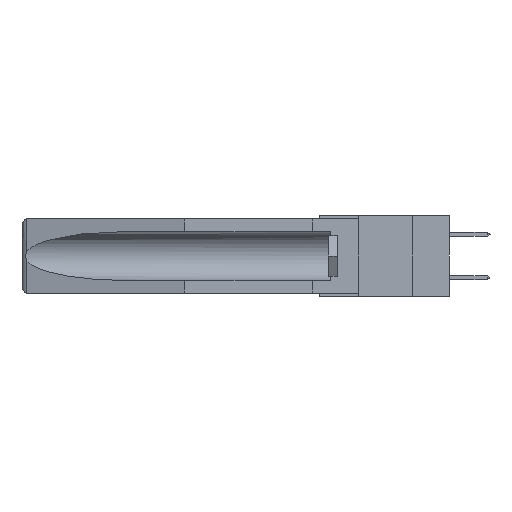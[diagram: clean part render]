
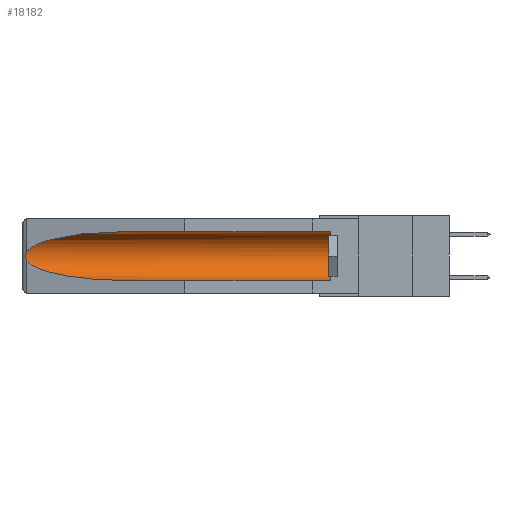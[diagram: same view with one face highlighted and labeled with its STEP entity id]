
A CAD part, left-side view. The second image highlights one B-rep face of the part: STEP entity #18182.
In plain terms, the highlighted cylindrical face has radius 2.857 mm (diameter 5.715 mm), a partial arc.
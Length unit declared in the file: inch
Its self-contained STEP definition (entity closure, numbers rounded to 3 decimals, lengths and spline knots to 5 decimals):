
#367 = ORIENTED_EDGE ( 'NONE', *, *, #15120, .T. ) ;
#2847 = LINE ( 'NONE', #16621, #24788 ) ;
#3473 = VERTEX_POINT ( 'NONE', #22331 ) ;
#3673 = EDGE_CURVE ( 'NONE', #22735, #22825, #7469, .T. ) ;
#3933 = CARTESIAN_POINT ( 'NONE',  ( 0.155, 0.126, -0.059 ) ) ;
#4370 = CARTESIAN_POINT ( 'NONE',  ( 0.155, 1.07973, -0.284 ) ) ;
#5345 = CARTESIAN_POINT ( 'NONE',  ( 0.26537, 1.52718, -0.19328 ) ) ;
#5605 = AXIS2_PLACEMENT_3D ( 'NONE', #23266, #19071, #17118 ) ;
#5941 = DIRECTION ( 'NONE',  ( 0., 1., 0. ) ) ;
#6650 = B_SPLINE_CURVE_WITH_KNOTS ( 'NONE', 3,
 ( #11245, #21569, #26173, #9099, #17680, #6893, #13090, #9195, #11066, #13365 ),
 .UNSPECIFIED., .F., .F.,
 ( 4, 2, 2, 2, 4 ),
 ( 0., 0.00029, 0.00058, 0.00087, 0.00117 ),
 .UNSPECIFIED. ) ;
#6893 = CARTESIAN_POINT ( 'NONE',  ( 0.2675, 1.53308, -0.17534 ) ) ;
#7223 = CYLINDRICAL_SURFACE ( 'NONE', #5605, 0.1125 ) ;
#7469 =( BOUNDED_CURVE ( )  B_SPLINE_CURVE ( 3, ( #10712, #19004, #23375, #14985 ),
 .UNSPECIFIED., .F., .F. ) 
 B_SPLINE_CURVE_WITH_KNOTS ( ( 4, 4 ),
 ( 4.71239, 6.08839 ),
 .UNSPECIFIED. ) 
 CURVE ( )  GEOMETRIC_REPRESENTATION_ITEM ( )  RATIONAL_B_SPLINE_CURVE ( ( 1., 0.848, 0.848, 1. ) ) 
 REPRESENTATION_ITEM ( '' )  );
#7756 = VERTEX_POINT ( 'NONE', #3933 ) ;
#8251 = EDGE_CURVE ( 'NONE', #7756, #22735, #2847, .T. ) ;
#8991 = EDGE_CURVE ( 'NONE', #22825, #3473, #6650, .T. ) ;
#9099 = CARTESIAN_POINT ( 'NONE',  ( 0.2673, 1.5327, -0.16383 ) ) ;
#9195 = CARTESIAN_POINT ( 'NONE',  ( 0.26655, 1.53094, -0.18657 ) ) ;
#10554 = ORIENTED_EDGE ( 'NONE', *, *, #3673, .T. ) ;
#10712 = CARTESIAN_POINT ( 'NONE',  ( 0.155, 1.07973, -0.059 ) ) ;
#11066 = CARTESIAN_POINT ( 'NONE',  ( 0.26597, 1.5296, -0.19026 ) ) ;
#11245 = CARTESIAN_POINT ( 'NONE',  ( 0.26537, 1.52718, -0.14972 ) ) ;
#12961 = EDGE_LOOP ( 'NONE', ( #10554, #13320, #367, #12995, #19176, #27422 ) ) ;
#12995 = ORIENTED_EDGE ( 'NONE', *, *, #15663, .F. ) ;
#13090 = CARTESIAN_POINT ( 'NONE',  ( 0.2673, 1.53269, -0.17917 ) ) ;
#13320 = ORIENTED_EDGE ( 'NONE', *, *, #8991, .T. ) ;
#13365 = CARTESIAN_POINT ( 'NONE',  ( 0.26537, 1.52718, -0.19328 ) ) ;
#13587 = DIRECTION ( 'NONE',  ( 0., -1., 0. ) ) ;
#13748 = CARTESIAN_POINT ( 'NONE',  ( 0.21114, 1.30732, -0.284 ) ) ;
#14320 = DIRECTION ( 'NONE',  ( 0., 1., 0. ) ) ;
#14541 = CARTESIAN_POINT ( 'NONE',  ( 0.155, 1.07973, -0.059 ) ) ;
#14985 = CARTESIAN_POINT ( 'NONE',  ( 0.26537, 1.52718, -0.14972 ) ) ;
#15120 = EDGE_CURVE ( 'NONE', #3473, #26263, #18226, .T. ) ;
#15663 = EDGE_CURVE ( 'NONE', #26857, #26263, #24049, .T. ) ;
#15803 = CARTESIAN_POINT ( 'NONE',  ( 0.25451, 1.48313, -0.24835 ) ) ;
#16184 = CIRCLE ( 'NONE', #21618, 0.1125 ) ;
#16621 = CARTESIAN_POINT ( 'NONE',  ( 0.155, -0.30754, -0.059 ) ) ;
#17118 = DIRECTION ( 'NONE',  ( 0., 0., 1. ) ) ;
#17680 = CARTESIAN_POINT ( 'NONE',  ( 0.2675, 1.53308, -0.16763 ) ) ;
#18182 = ADVANCED_FACE ( 'NONE', ( #26260 ), #7223, .F. ) ;
#18226 =( BOUNDED_CURVE ( )  B_SPLINE_CURVE ( 3, ( #5345, #15803, #13748, #20175 ),
 .UNSPECIFIED., .F., .T. ) 
 B_SPLINE_CURVE_WITH_KNOTS ( ( 4, 4 ),
 ( 0.1948, 1.5708 ),
 .UNSPECIFIED. ) 
 CURVE ( )  GEOMETRIC_REPRESENTATION_ITEM ( )  RATIONAL_B_SPLINE_CURVE ( ( 1., 0.848, 0.848, 1. ) ) 
 REPRESENTATION_ITEM ( '' )  );
#18388 = VECTOR ( 'NONE', #14320, 39.37008 ) ;
#18502 = EDGE_CURVE ( 'NONE', #26857, #7756, #16184, .T. ) ;
#19004 = CARTESIAN_POINT ( 'NONE',  ( 0.21114, 1.30732, -0.059 ) ) ;
#19071 = DIRECTION ( 'NONE',  ( 0., 1., 0. ) ) ;
#19176 = ORIENTED_EDGE ( 'NONE', *, *, #18502, .T. ) ;
#20175 = CARTESIAN_POINT ( 'NONE',  ( 0.155, 1.07973, -0.284 ) ) ;
#20975 = CARTESIAN_POINT ( 'NONE',  ( 0.155, -0.30754, -0.284 ) ) ;
#21217 = CARTESIAN_POINT ( 'NONE',  ( 0.26537, 1.52718, -0.14972 ) ) ;
#21569 = CARTESIAN_POINT ( 'NONE',  ( 0.26597, 1.52961, -0.15275 ) ) ;
#21618 = AXIS2_PLACEMENT_3D ( 'NONE', #24516, #13587, #24324 ) ;
#22331 = CARTESIAN_POINT ( 'NONE',  ( 0.26537, 1.52718, -0.19328 ) ) ;
#22735 = VERTEX_POINT ( 'NONE', #14541 ) ;
#22825 = VERTEX_POINT ( 'NONE', #21217 ) ;
#23266 = CARTESIAN_POINT ( 'NONE',  ( 0.155, -0.30754, -0.1715 ) ) ;
#23375 = CARTESIAN_POINT ( 'NONE',  ( 0.25451, 1.48313, -0.09465 ) ) ;
#24049 = LINE ( 'NONE', #20975, #18388 ) ;
#24324 = DIRECTION ( 'NONE',  ( 0., 0., 1. ) ) ;
#24516 = CARTESIAN_POINT ( 'NONE',  ( 0.155, 0.126, -0.1715 ) ) ;
#24788 = VECTOR ( 'NONE', #5941, 39.37008 ) ;
#26173 = CARTESIAN_POINT ( 'NONE',  ( 0.26654, 1.53092, -0.15636 ) ) ;
#26260 = FACE_OUTER_BOUND ( 'NONE', #12961, .T. ) ;
#26263 = VERTEX_POINT ( 'NONE', #4370 ) ;
#26857 = VERTEX_POINT ( 'NONE', #27210 ) ;
#27210 = CARTESIAN_POINT ( 'NONE',  ( 0.155, 0.126, -0.284 ) ) ;
#27422 = ORIENTED_EDGE ( 'NONE', *, *, #8251, .T. ) ;
